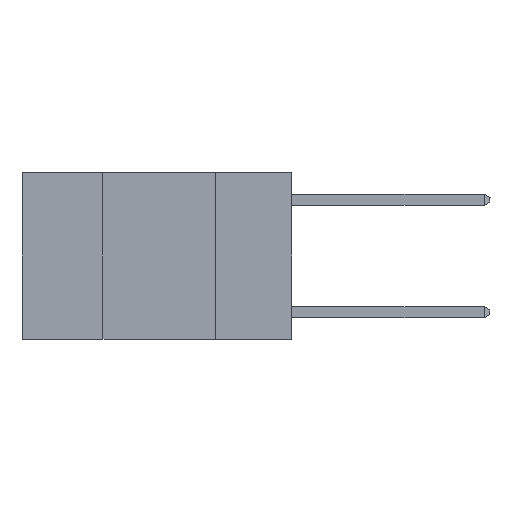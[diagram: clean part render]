
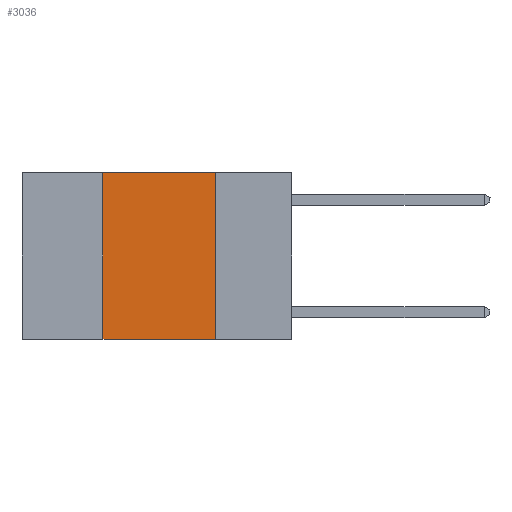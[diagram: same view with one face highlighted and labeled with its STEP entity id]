
A CAD part, left-side view. The second image highlights one B-rep face of the part: STEP entity #3036.
In plain terms, the highlighted planar face has unit normal (-1, 0, 0).
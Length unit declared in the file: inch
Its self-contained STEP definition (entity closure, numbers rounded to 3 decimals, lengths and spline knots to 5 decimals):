
#635 = CARTESIAN_POINT ( 'NONE',  ( 0., 0.6, -0.37 ) ) ;
#1106 = AXIS2_PLACEMENT_3D ( 'NONE', #23154, #19352, #20901 ) ;
#2008 = VERTEX_POINT ( 'NONE', #12640 ) ;
#2228 = FACE_OUTER_BOUND ( 'NONE', #11400, .T. ) ;
#2621 = CARTESIAN_POINT ( 'NONE',  ( 0., 0.17, 0. ) ) ;
#3022 = LINE ( 'NONE', #635, #15854 ) ;
#3036 = ADVANCED_FACE ( 'NONE', ( #2228 ), #6140, .F. ) ;
#3403 = CARTESIAN_POINT ( 'NONE',  ( 0., 0.6, 0. ) ) ;
#4256 = VECTOR ( 'NONE', #8562, 39.37008 ) ;
#4599 = CARTESIAN_POINT ( 'NONE',  ( 0., 0.42, 0. ) ) ;
#4675 = VECTOR ( 'NONE', #4974, 39.37008 ) ;
#4974 = DIRECTION ( 'NONE',  ( 0., 0., 1. ) ) ;
#6140 = PLANE ( 'NONE',  #1106 ) ;
#8346 = DIRECTION ( 'NONE',  ( 0., -1., 0. ) ) ;
#8562 = DIRECTION ( 'NONE',  ( 0., 0., -1. ) ) ;
#9052 = EDGE_CURVE ( 'NONE', #10301, #20338, #3022, .T. ) ;
#10301 = VERTEX_POINT ( 'NONE', #16131 ) ;
#10393 = VECTOR ( 'NONE', #20933, 39.37008 ) ;
#10728 = LINE ( 'NONE', #20087, #4675 ) ;
#11023 = ORIENTED_EDGE ( 'NONE', *, *, #9052, .T. ) ;
#11150 = CARTESIAN_POINT ( 'NONE',  ( 0., 0.17, -0.37 ) ) ;
#11400 = EDGE_LOOP ( 'NONE', ( #13850, #16314, #20056, #11023 ) ) ;
#12640 = CARTESIAN_POINT ( 'NONE',  ( 0., 0.17, 0. ) ) ;
#13850 = ORIENTED_EDGE ( 'NONE', *, *, #17094, .F. ) ;
#15854 = VECTOR ( 'NONE', #8346, 39.37008 ) ;
#15995 = VERTEX_POINT ( 'NONE', #4599 ) ;
#16131 = CARTESIAN_POINT ( 'NONE',  ( 0., 0.42, -0.37 ) ) ;
#16314 = ORIENTED_EDGE ( 'NONE', *, *, #24281, .F. ) ;
#17094 = EDGE_CURVE ( 'NONE', #2008, #20338, #21553, .T. ) ;
#19352 = DIRECTION ( 'NONE',  ( 1., 0., 0. ) ) ;
#19493 = EDGE_CURVE ( 'NONE', #10301, #15995, #10728, .T. ) ;
#20056 = ORIENTED_EDGE ( 'NONE', *, *, #19493, .F. ) ;
#20087 = CARTESIAN_POINT ( 'NONE',  ( 0., 0.42, 0. ) ) ;
#20338 = VERTEX_POINT ( 'NONE', #11150 ) ;
#20901 = DIRECTION ( 'NONE',  ( 0., 0., -1. ) ) ;
#20933 = DIRECTION ( 'NONE',  ( 0., -1., 0. ) ) ;
#21553 = LINE ( 'NONE', #2621, #4256 ) ;
#23154 = CARTESIAN_POINT ( 'NONE',  ( 0., 0.6, 0. ) ) ;
#24281 = EDGE_CURVE ( 'NONE', #15995, #2008, #24703, .T. ) ;
#24703 = LINE ( 'NONE', #3403, #10393 ) ;
